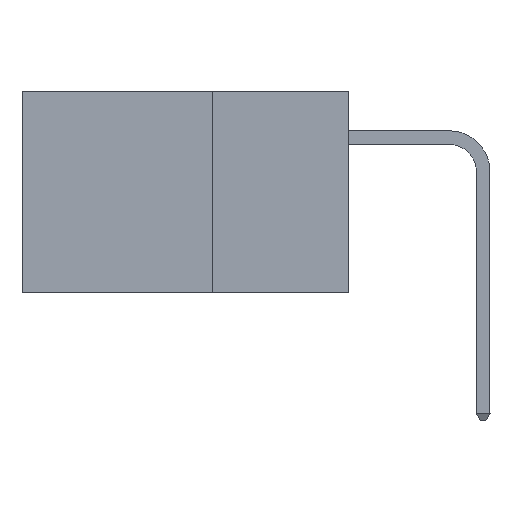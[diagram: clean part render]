
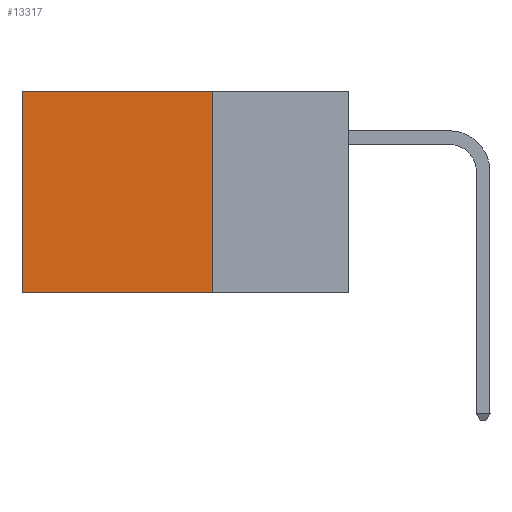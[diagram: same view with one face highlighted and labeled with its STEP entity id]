
A CAD part, left-side view. The second image highlights one B-rep face of the part: STEP entity #13317.
In plain terms, the highlighted planar face has unit normal (-1, 0, 0).
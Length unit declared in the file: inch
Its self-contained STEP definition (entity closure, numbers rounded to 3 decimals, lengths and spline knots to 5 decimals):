
#1299 = PLANE ( 'NONE',  #1767 ) ;
#1767 = AXIS2_PLACEMENT_3D ( 'NONE', #43496, #32775, #15213 ) ;
#2104 = VECTOR ( 'NONE', #5503, 39.37008 ) ;
#2529 = LINE ( 'NONE', #23737, #2104 ) ;
#3503 = VECTOR ( 'NONE', #17604, 39.37008 ) ;
#4398 = CARTESIAN_POINT ( 'NONE',  ( 0.2875, 0.25, -0.37 ) ) ;
#5161 = CARTESIAN_POINT ( 'NONE',  ( 0.2875, 0.25, 0. ) ) ;
#5503 = DIRECTION ( 'NONE',  ( 0., 0., -1. ) ) ;
#11222 = LINE ( 'NONE', #34946, #3503 ) ;
#13317 = ADVANCED_FACE ( 'NONE', ( #32553 ), #1299, .F. ) ;
#15213 = DIRECTION ( 'NONE',  ( 0., 0., -1. ) ) ;
#15988 = EDGE_CURVE ( 'NONE', #34352, #22907, #36406, .T. ) ;
#17159 = EDGE_CURVE ( 'NONE', #31073, #26592, #2529, .T. ) ;
#17604 = DIRECTION ( 'NONE',  ( 0., 1., 0. ) ) ;
#19073 = DIRECTION ( 'NONE',  ( 0., 0., -1. ) ) ;
#22672 = CARTESIAN_POINT ( 'NONE',  ( 0.2875, 0.25, 0. ) ) ;
#22907 = VERTEX_POINT ( 'NONE', #4398 ) ;
#23697 = LINE ( 'NONE', #26672, #40406 ) ;
#23737 = CARTESIAN_POINT ( 'NONE',  ( 0.2875, 0.6, 0. ) ) ;
#25340 = ORIENTED_EDGE ( 'NONE', *, *, #17159, .T. ) ;
#25461 = EDGE_LOOP ( 'NONE', ( #25340, #31448, #35139, #40547 ) ) ;
#26592 = VERTEX_POINT ( 'NONE', #28579 ) ;
#26672 = CARTESIAN_POINT ( 'NONE',  ( 0.2875, 0.25, 0. ) ) ;
#28579 = CARTESIAN_POINT ( 'NONE',  ( 0.2875, 0.6, -0.37 ) ) ;
#29014 = VECTOR ( 'NONE', #19073, 39.37008 ) ;
#30532 = DIRECTION ( 'NONE',  ( 0., 1., 0. ) ) ;
#31073 = VERTEX_POINT ( 'NONE', #39468 ) ;
#31448 = ORIENTED_EDGE ( 'NONE', *, *, #42324, .F. ) ;
#32553 = FACE_OUTER_BOUND ( 'NONE', #25461, .T. ) ;
#32775 = DIRECTION ( 'NONE',  ( 1., 0., 0. ) ) ;
#34352 = VERTEX_POINT ( 'NONE', #22672 ) ;
#34946 = CARTESIAN_POINT ( 'NONE',  ( 0.2875, 0.25, -0.37 ) ) ;
#35139 = ORIENTED_EDGE ( 'NONE', *, *, #15988, .F. ) ;
#36406 = LINE ( 'NONE', #5161, #29014 ) ;
#36627 = EDGE_CURVE ( 'NONE', #34352, #31073, #23697, .T. ) ;
#39468 = CARTESIAN_POINT ( 'NONE',  ( 0.2875, 0.6, 0. ) ) ;
#40406 = VECTOR ( 'NONE', #30532, 39.37008 ) ;
#40547 = ORIENTED_EDGE ( 'NONE', *, *, #36627, .T. ) ;
#42324 = EDGE_CURVE ( 'NONE', #22907, #26592, #11222, .T. ) ;
#43496 = CARTESIAN_POINT ( 'NONE',  ( 0.2875, 0.25, 0. ) ) ;
